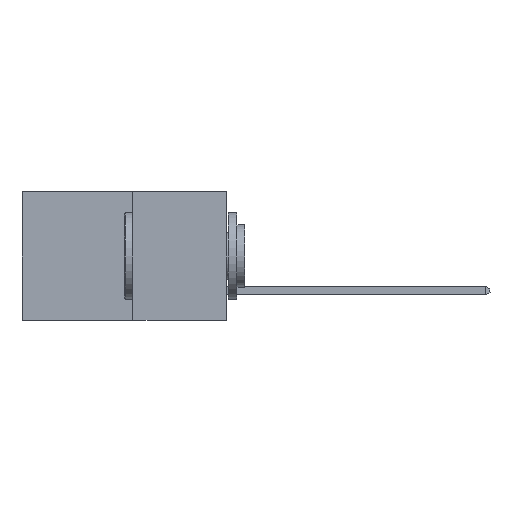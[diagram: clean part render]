
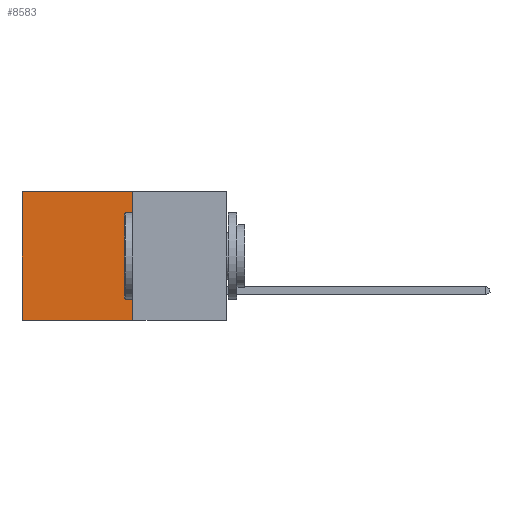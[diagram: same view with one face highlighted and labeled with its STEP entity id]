
A CAD part, left-side view. The second image highlights one B-rep face of the part: STEP entity #8583.
In plain terms, the highlighted planar face has unit normal (-1, 0, 0).
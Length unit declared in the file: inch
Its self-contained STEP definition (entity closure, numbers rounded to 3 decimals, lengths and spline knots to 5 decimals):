
#16 = VERTEX_POINT ( 'NONE', #7885 ) ;
#175 = CARTESIAN_POINT ( 'NONE',  ( 0.277, 0.27, -0.37 ) ) ;
#316 = VECTOR ( 'NONE', #1171, 39.37008 ) ;
#1117 = CARTESIAN_POINT ( 'NONE',  ( 0.277, 0.59, -0.37 ) ) ;
#1171 = DIRECTION ( 'NONE',  ( 0., 0., -1. ) ) ;
#1866 = VECTOR ( 'NONE', #10661, 39.37008 ) ;
#1962 = ORIENTED_EDGE ( 'NONE', *, *, #7615, .F. ) ;
#2028 = CARTESIAN_POINT ( 'NONE',  ( 0.277, 0.27, -0.37 ) ) ;
#2125 = LINE ( 'NONE', #2715, #11987 ) ;
#2379 = VERTEX_POINT ( 'NONE', #5669 ) ;
#2715 = CARTESIAN_POINT ( 'NONE',  ( 0.277, 0.27, -0.37 ) ) ;
#3508 = PLANE ( 'NONE',  #7125 ) ;
#4035 = EDGE_CURVE ( 'NONE', #16, #2379, #10494, .T. ) ;
#4102 = VERTEX_POINT ( 'NONE', #12443 ) ;
#4393 = ORIENTED_EDGE ( 'NONE', *, *, #7866, .F. ) ;
#4530 = DIRECTION ( 'NONE',  ( 0., 0., -1. ) ) ;
#4563 = FACE_OUTER_BOUND ( 'NONE', #10721, .T. ) ;
#5504 = CARTESIAN_POINT ( 'NONE',  ( 0.277, 0.27, -0.37 ) ) ;
#5669 = CARTESIAN_POINT ( 'NONE',  ( 0.277, 0.59, -0.37 ) ) ;
#6104 = EDGE_CURVE ( 'NONE', #4102, #16, #7216, .T. ) ;
#6425 = DIRECTION ( 'NONE',  ( 0., 0., -1. ) ) ;
#7125 = AXIS2_PLACEMENT_3D ( 'NONE', #5504, #10166, #4530 ) ;
#7216 = LINE ( 'NONE', #9773, #1866 ) ;
#7615 = EDGE_CURVE ( 'NONE', #4102, #9015, #11575, .T. ) ;
#7866 = EDGE_CURVE ( 'NONE', #9015, #2379, #2125, .T. ) ;
#7885 = CARTESIAN_POINT ( 'NONE',  ( 0.277, 0.59, 0. ) ) ;
#8583 = ADVANCED_FACE ( 'NONE', ( #4563 ), #3508, .F. ) ;
#9015 = VERTEX_POINT ( 'NONE', #2028 ) ;
#9191 = ORIENTED_EDGE ( 'NONE', *, *, #4035, .T. ) ;
#9209 = VECTOR ( 'NONE', #6425, 39.37008 ) ;
#9773 = CARTESIAN_POINT ( 'NONE',  ( 0.277, 0.27, 0. ) ) ;
#10166 = DIRECTION ( 'NONE',  ( 1., 0., 0. ) ) ;
#10301 = ORIENTED_EDGE ( 'NONE', *, *, #6104, .T. ) ;
#10383 = DIRECTION ( 'NONE',  ( 0., 1., 0. ) ) ;
#10494 = LINE ( 'NONE', #1117, #316 ) ;
#10661 = DIRECTION ( 'NONE',  ( 0., 1., 0. ) ) ;
#10721 = EDGE_LOOP ( 'NONE', ( #9191, #4393, #1962, #10301 ) ) ;
#11575 = LINE ( 'NONE', #175, #9209 ) ;
#11987 = VECTOR ( 'NONE', #10383, 39.37008 ) ;
#12443 = CARTESIAN_POINT ( 'NONE',  ( 0.277, 0.27, 0. ) ) ;
